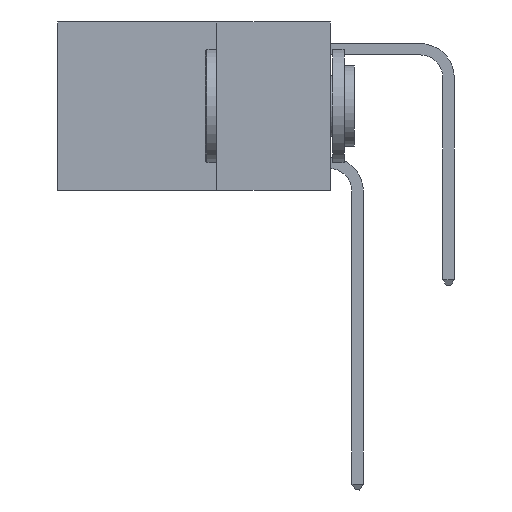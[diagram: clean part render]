
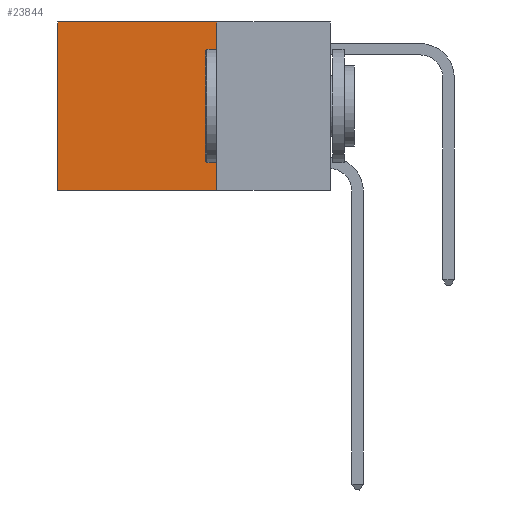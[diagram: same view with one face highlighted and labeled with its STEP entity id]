
A CAD part, left-side view. The second image highlights one B-rep face of the part: STEP entity #23844.
In plain terms, the highlighted planar face has unit normal (-1, 0, 0).
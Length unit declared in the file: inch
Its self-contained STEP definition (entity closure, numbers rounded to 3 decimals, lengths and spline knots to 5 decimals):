
#129 = VECTOR ( 'NONE', #18652, 39.37008 ) ;
#462 = VERTEX_POINT ( 'NONE', #25631 ) ;
#888 = CARTESIAN_POINT ( 'NONE',  ( 0.2625, 0.6, 0. ) ) ;
#971 = ORIENTED_EDGE ( 'NONE', *, *, #4945, .T. ) ;
#1316 = CARTESIAN_POINT ( 'NONE',  ( 0.2625, 0.6, 0. ) ) ;
#2679 = VERTEX_POINT ( 'NONE', #15681 ) ;
#4405 = DIRECTION ( 'NONE',  ( 0., 1., 0. ) ) ;
#4945 = EDGE_CURVE ( 'NONE', #20457, #2679, #11516, .T. ) ;
#5027 = ORIENTED_EDGE ( 'NONE', *, *, #14331, .F. ) ;
#5128 = FACE_OUTER_BOUND ( 'NONE', #7025, .T. ) ;
#5265 = VECTOR ( 'NONE', #16480, 39.37008 ) ;
#5854 = CARTESIAN_POINT ( 'NONE',  ( 0.2625, 0.25, 0. ) ) ;
#6348 = CARTESIAN_POINT ( 'NONE',  ( 0.2625, 0.25, 0. ) ) ;
#7025 = EDGE_LOOP ( 'NONE', ( #971, #28898, #5027, #11079 ) ) ;
#8430 = DIRECTION ( 'NONE',  ( 1., 0., 0. ) ) ;
#10102 = CARTESIAN_POINT ( 'NONE',  ( 0.2625, 0.25, 0. ) ) ;
#10571 = PLANE ( 'NONE',  #19306 ) ;
#10638 = VECTOR ( 'NONE', #15006, 39.37008 ) ;
#11079 = ORIENTED_EDGE ( 'NONE', *, *, #20701, .T. ) ;
#11516 = LINE ( 'NONE', #1316, #5265 ) ;
#14331 = EDGE_CURVE ( 'NONE', #462, #25602, #20901, .T. ) ;
#14827 = VECTOR ( 'NONE', #4405, 39.37008 ) ;
#15006 = DIRECTION ( 'NONE',  ( 0., 0., -1. ) ) ;
#15681 = CARTESIAN_POINT ( 'NONE',  ( 0.2625, 0.6, -0.37 ) ) ;
#16284 = LINE ( 'NONE', #18549, #129 ) ;
#16480 = DIRECTION ( 'NONE',  ( 0., 0., -1. ) ) ;
#17665 = EDGE_CURVE ( 'NONE', #25602, #2679, #16284, .T. ) ;
#18549 = CARTESIAN_POINT ( 'NONE',  ( 0.2625, 0.25, -0.37 ) ) ;
#18652 = DIRECTION ( 'NONE',  ( 0., 1., 0. ) ) ;
#19306 = AXIS2_PLACEMENT_3D ( 'NONE', #5854, #8430, #19968 ) ;
#19968 = DIRECTION ( 'NONE',  ( 0., 0., -1. ) ) ;
#20457 = VERTEX_POINT ( 'NONE', #888 ) ;
#20701 = EDGE_CURVE ( 'NONE', #462, #20457, #24385, .T. ) ;
#20901 = LINE ( 'NONE', #10102, #10638 ) ;
#23537 = CARTESIAN_POINT ( 'NONE',  ( 0.2625, 0.25, -0.37 ) ) ;
#23844 = ADVANCED_FACE ( 'NONE', ( #5128 ), #10571, .F. ) ;
#24385 = LINE ( 'NONE', #6348, #14827 ) ;
#25602 = VERTEX_POINT ( 'NONE', #23537 ) ;
#25631 = CARTESIAN_POINT ( 'NONE',  ( 0.2625, 0.25, 0. ) ) ;
#28898 = ORIENTED_EDGE ( 'NONE', *, *, #17665, .F. ) ;
